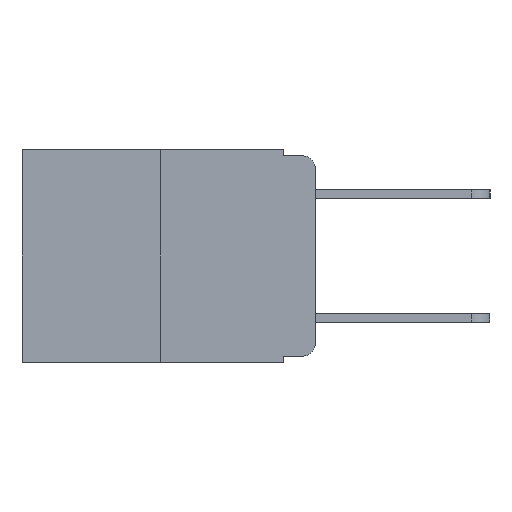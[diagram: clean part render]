
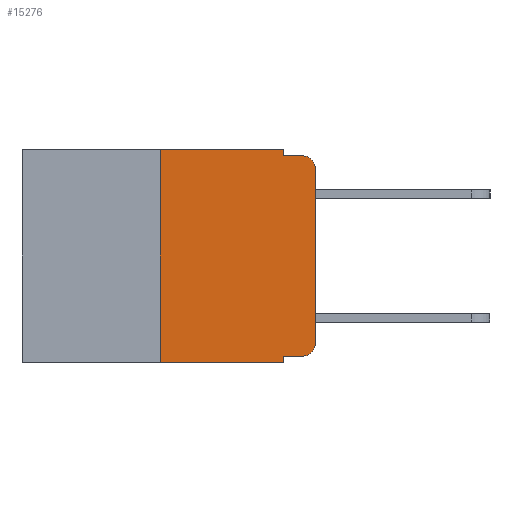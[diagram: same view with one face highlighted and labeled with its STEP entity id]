
A CAD part, left-side view. The second image highlights one B-rep face of the part: STEP entity #15276.
In plain terms, the highlighted planar face has unit normal (-1, 0, 0).
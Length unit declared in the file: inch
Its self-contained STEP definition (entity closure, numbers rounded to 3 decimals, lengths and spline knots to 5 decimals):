
#108 = CARTESIAN_POINT ( 'NONE',  ( 0., 0.051, -0.333 ) ) ;
#362 = CARTESIAN_POINT ( 'NONE',  ( 0., 0.25, 0. ) ) ;
#448 = AXIS2_PLACEMENT_3D ( 'NONE', #13582, #13577, #13003 ) ;
#732 = LINE ( 'NONE', #108, #4631 ) ;
#777 = VECTOR ( 'NONE', #17808, 39.37008 ) ;
#943 = LINE ( 'NONE', #7794, #16302 ) ;
#1695 = FACE_OUTER_BOUND ( 'NONE', #5420, .T. ) ;
#1755 = VECTOR ( 'NONE', #16236, 39.37008 ) ;
#1993 = VERTEX_POINT ( 'NONE', #14676 ) ;
#2032 = CARTESIAN_POINT ( 'NONE',  ( 0., 0.051, 0. ) ) ;
#2190 = ORIENTED_EDGE ( 'NONE', *, *, #5837, .F. ) ;
#2224 = DIRECTION ( 'NONE',  ( 1., 0., 0. ) ) ;
#2454 = VERTEX_POINT ( 'NONE', #2726 ) ;
#2509 = EDGE_CURVE ( 'NONE', #3967, #3139, #10454, .T. ) ;
#2611 = CARTESIAN_POINT ( 'NONE',  ( 0., 0.051, -0.01 ) ) ;
#2710 = EDGE_CURVE ( 'NONE', #3482, #8240, #943, .T. ) ;
#2726 = CARTESIAN_POINT ( 'NONE',  ( 0., 0.051, -0.333 ) ) ;
#3139 = VERTEX_POINT ( 'NONE', #6568 ) ;
#3482 = VERTEX_POINT ( 'NONE', #11002 ) ;
#3528 = CARTESIAN_POINT ( 'NONE',  ( 0., 0., -0.03 ) ) ;
#3535 = LINE ( 'NONE', #14203, #7209 ) ;
#3792 = CIRCLE ( 'NONE', #448, 0.02 ) ;
#3813 = CARTESIAN_POINT ( 'NONE',  ( 0., 0.473, 0. ) ) ;
#3892 = EDGE_CURVE ( 'NONE', #11944, #7596, #3792, .T. ) ;
#3967 = VERTEX_POINT ( 'NONE', #3528 ) ;
#4214 = ORIENTED_EDGE ( 'NONE', *, *, #13088, .F. ) ;
#4631 = VECTOR ( 'NONE', #10944, 39.37008 ) ;
#4963 = ORIENTED_EDGE ( 'NONE', *, *, #2710, .T. ) ;
#5046 = LINE ( 'NONE', #362, #12405 ) ;
#5326 = DIRECTION ( 'NONE',  ( 0., 0., 1. ) ) ;
#5420 = EDGE_LOOP ( 'NONE', ( #12044, #12921, #14234, #15775, #2190, #4214, #4963, #5666, #7319, #7795 ) ) ;
#5600 = VECTOR ( 'NONE', #6845, 39.37008 ) ;
#5666 = ORIENTED_EDGE ( 'NONE', *, *, #11229, .F. ) ;
#5837 = EDGE_CURVE ( 'NONE', #1993, #14028, #9225, .T. ) ;
#6568 = CARTESIAN_POINT ( 'NONE',  ( 0., 0.02, -0.01 ) ) ;
#6635 = EDGE_CURVE ( 'NONE', #2454, #11944, #732, .T. ) ;
#6845 = DIRECTION ( 'NONE',  ( 0., 0., -1. ) ) ;
#6937 = VERTEX_POINT ( 'NONE', #2611 ) ;
#7188 = CARTESIAN_POINT ( 'NONE',  ( 0., 0.051, -0.01 ) ) ;
#7209 = VECTOR ( 'NONE', #8614, 39.37008 ) ;
#7319 = ORIENTED_EDGE ( 'NONE', *, *, #6635, .T. ) ;
#7596 = VERTEX_POINT ( 'NONE', #16086 ) ;
#7794 = CARTESIAN_POINT ( 'NONE',  ( 0., 0.473, -0.343 ) ) ;
#7795 = ORIENTED_EDGE ( 'NONE', *, *, #3892, .T. ) ;
#7962 = LINE ( 'NONE', #7188, #10477 ) ;
#8240 = VERTEX_POINT ( 'NONE', #8605 ) ;
#8515 = EDGE_CURVE ( 'NONE', #7596, #3967, #13698, .T. ) ;
#8605 = CARTESIAN_POINT ( 'NONE',  ( 0., 0.051, -0.343 ) ) ;
#8614 = DIRECTION ( 'NONE',  ( 0., 0., -1. ) ) ;
#9225 = LINE ( 'NONE', #17721, #777 ) ;
#9956 = PLANE ( 'NONE',  #16536 ) ;
#10454 = CIRCLE ( 'NONE', #16985, 0.02 ) ;
#10477 = VECTOR ( 'NONE', #18285, 39.37008 ) ;
#10944 = DIRECTION ( 'NONE',  ( 0., -1., 0. ) ) ;
#11002 = CARTESIAN_POINT ( 'NONE',  ( 0., 0.25, -0.343 ) ) ;
#11229 = EDGE_CURVE ( 'NONE', #2454, #8240, #13327, .T. ) ;
#11944 = VERTEX_POINT ( 'NONE', #14059 ) ;
#12019 = EDGE_CURVE ( 'NONE', #6937, #3139, #7962, .T. ) ;
#12044 = ORIENTED_EDGE ( 'NONE', *, *, #8515, .T. ) ;
#12405 = VECTOR ( 'NONE', #5326, 39.37008 ) ;
#12732 = DIRECTION ( 'NONE',  ( 0., 0., -1. ) ) ;
#12898 = DIRECTION ( 'NONE',  ( 0., -1., 0. ) ) ;
#12921 = ORIENTED_EDGE ( 'NONE', *, *, #2509, .T. ) ;
#13003 = DIRECTION ( 'NONE',  ( 0., 0., -1. ) ) ;
#13088 = EDGE_CURVE ( 'NONE', #3482, #1993, #5046, .T. ) ;
#13196 = EDGE_CURVE ( 'NONE', #14028, #6937, #3535, .T. ) ;
#13327 = LINE ( 'NONE', #2032, #5600 ) ;
#13577 = DIRECTION ( 'NONE',  ( -1., 0., 0. ) ) ;
#13582 = CARTESIAN_POINT ( 'NONE',  ( 0., 0.02, -0.313 ) ) ;
#13698 = LINE ( 'NONE', #16178, #1755 ) ;
#14028 = VERTEX_POINT ( 'NONE', #15639 ) ;
#14059 = CARTESIAN_POINT ( 'NONE',  ( 0., 0.02, -0.333 ) ) ;
#14203 = CARTESIAN_POINT ( 'NONE',  ( 0., 0.051, 0. ) ) ;
#14234 = ORIENTED_EDGE ( 'NONE', *, *, #12019, .F. ) ;
#14676 = CARTESIAN_POINT ( 'NONE',  ( 0., 0.25, 0. ) ) ;
#15272 = DIRECTION ( 'NONE',  ( 0., 0., -1. ) ) ;
#15276 = ADVANCED_FACE ( 'NONE', ( #1695 ), #9956, .F. ) ;
#15588 = CARTESIAN_POINT ( 'NONE',  ( 0., 0.02, -0.03 ) ) ;
#15639 = CARTESIAN_POINT ( 'NONE',  ( 0., 0.051, 0. ) ) ;
#15775 = ORIENTED_EDGE ( 'NONE', *, *, #13196, .F. ) ;
#16086 = CARTESIAN_POINT ( 'NONE',  ( 0., 0., -0.313 ) ) ;
#16178 = CARTESIAN_POINT ( 'NONE',  ( 0., 0., 0. ) ) ;
#16236 = DIRECTION ( 'NONE',  ( 0., 0., 1. ) ) ;
#16302 = VECTOR ( 'NONE', #12898, 39.37008 ) ;
#16367 = DIRECTION ( 'NONE',  ( -1., 0., 0. ) ) ;
#16536 = AXIS2_PLACEMENT_3D ( 'NONE', #3813, #2224, #12732 ) ;
#16985 = AXIS2_PLACEMENT_3D ( 'NONE', #15588, #16367, #15272 ) ;
#17721 = CARTESIAN_POINT ( 'NONE',  ( 0., 0.473, 0. ) ) ;
#17808 = DIRECTION ( 'NONE',  ( 0., -1., 0. ) ) ;
#18285 = DIRECTION ( 'NONE',  ( 0., -1., 0. ) ) ;
